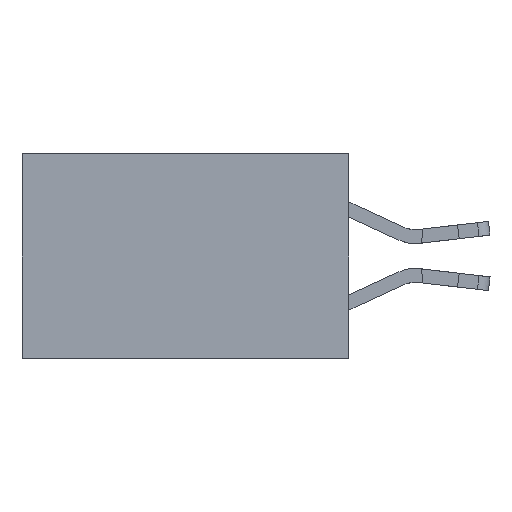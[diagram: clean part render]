
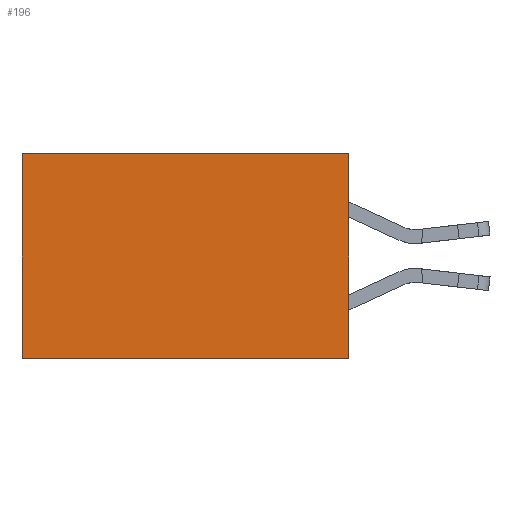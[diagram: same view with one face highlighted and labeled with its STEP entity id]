
A CAD part, left-side view. The second image highlights one B-rep face of the part: STEP entity #196.
In plain terms, the highlighted planar face has unit normal (-1, 0, 0).
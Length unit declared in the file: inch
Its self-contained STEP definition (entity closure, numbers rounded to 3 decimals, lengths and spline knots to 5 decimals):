
#196 = ADVANCED_FACE ( 'NONE', ( #813 ), #8492, .F. ) ;
#248 = VECTOR ( 'NONE', #16893, 39.37008 ) ;
#768 = CARTESIAN_POINT ( 'NONE',  ( 0.277, 0., -0.37 ) ) ;
#813 = FACE_OUTER_BOUND ( 'NONE', #5063, .T. ) ;
#1547 = CARTESIAN_POINT ( 'NONE',  ( 0.277, 0., 0. ) ) ;
#1907 = VECTOR ( 'NONE', #20192, 39.37008 ) ;
#2226 = ORIENTED_EDGE ( 'NONE', *, *, #19708, .F. ) ;
#2258 = ORIENTED_EDGE ( 'NONE', *, *, #18788, .T. ) ;
#3665 = VERTEX_POINT ( 'NONE', #5639 ) ;
#3734 = DIRECTION ( 'NONE',  ( 0., 0., -1. ) ) ;
#4727 = CARTESIAN_POINT ( 'NONE',  ( 0.277, 0.59, -0.37 ) ) ;
#5063 = EDGE_LOOP ( 'NONE', ( #17968, #17419, #2226, #2258 ) ) ;
#5639 = CARTESIAN_POINT ( 'NONE',  ( 0.277, 0.59, -0.37 ) ) ;
#5660 = CARTESIAN_POINT ( 'NONE',  ( 0.277, 0., -0.37 ) ) ;
#5892 = VERTEX_POINT ( 'NONE', #7444 ) ;
#7444 = CARTESIAN_POINT ( 'NONE',  ( 0.277, 0.59, 0. ) ) ;
#7828 = EDGE_CURVE ( 'NONE', #13209, #3665, #20602, .T. ) ;
#8422 = VECTOR ( 'NONE', #14725, 39.37008 ) ;
#8437 = DIRECTION ( 'NONE',  ( 1., 0., 0. ) ) ;
#8483 = DIRECTION ( 'NONE',  ( 0., 0., -1. ) ) ;
#8492 = PLANE ( 'NONE',  #10350 ) ;
#9286 = EDGE_CURVE ( 'NONE', #5892, #3665, #20095, .T. ) ;
#10350 = AXIS2_PLACEMENT_3D ( 'NONE', #5660, #8437, #8483 ) ;
#11753 = VECTOR ( 'NONE', #3734, 39.37008 ) ;
#12790 = LINE ( 'NONE', #1547, #8422 ) ;
#13209 = VERTEX_POINT ( 'NONE', #768 ) ;
#14725 = DIRECTION ( 'NONE',  ( 0., 1., 0. ) ) ;
#15405 = CARTESIAN_POINT ( 'NONE',  ( 0.277, 0., 0. ) ) ;
#15538 = LINE ( 'NONE', #18691, #1907 ) ;
#16893 = DIRECTION ( 'NONE',  ( 0., 1., 0. ) ) ;
#17079 = CARTESIAN_POINT ( 'NONE',  ( 0.277, 0., -0.37 ) ) ;
#17419 = ORIENTED_EDGE ( 'NONE', *, *, #7828, .F. ) ;
#17968 = ORIENTED_EDGE ( 'NONE', *, *, #9286, .T. ) ;
#18691 = CARTESIAN_POINT ( 'NONE',  ( 0.277, 0., -0.37 ) ) ;
#18788 = EDGE_CURVE ( 'NONE', #19069, #5892, #12790, .T. ) ;
#19069 = VERTEX_POINT ( 'NONE', #15405 ) ;
#19708 = EDGE_CURVE ( 'NONE', #19069, #13209, #15538, .T. ) ;
#20095 = LINE ( 'NONE', #4727, #11753 ) ;
#20192 = DIRECTION ( 'NONE',  ( 0., 0., -1. ) ) ;
#20602 = LINE ( 'NONE', #17079, #248 ) ;
